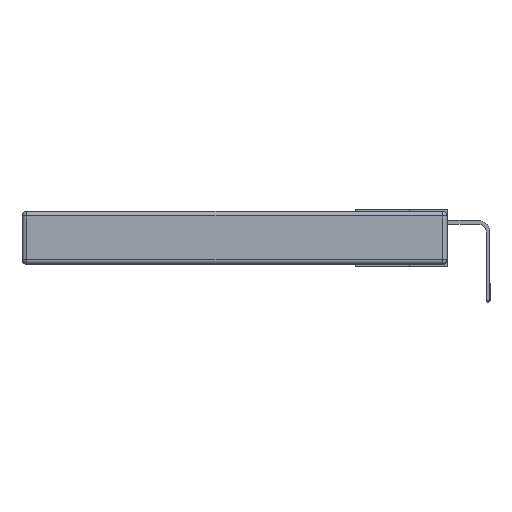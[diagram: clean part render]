
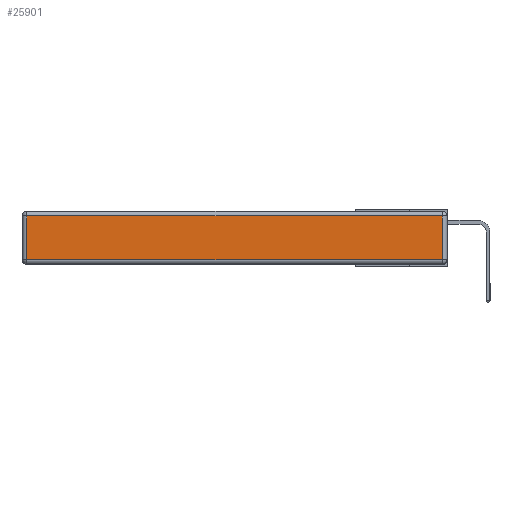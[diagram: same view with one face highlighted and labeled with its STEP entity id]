
A CAD part, left-side view. The second image highlights one B-rep face of the part: STEP entity #25901.
In plain terms, the highlighted planar face has unit normal (-1, 0, 0).
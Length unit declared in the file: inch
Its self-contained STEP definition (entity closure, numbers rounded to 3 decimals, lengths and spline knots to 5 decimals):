
#17 = EDGE_LOOP ( 'NONE', ( #25695, #3863, #17642, #13371 ) ) ;
#898 = VECTOR ( 'NONE', #26544, 39.37008 ) ;
#928 = VECTOR ( 'NONE', #22394, 39.37008 ) ;
#1292 = EDGE_CURVE ( 'NONE', #3934, #8542, #13863, .T. ) ;
#2066 = LINE ( 'NONE', #24042, #22711 ) ;
#2088 = EDGE_CURVE ( 'NONE', #15736, #11245, #26058, .T. ) ;
#3447 = LINE ( 'NONE', #5384, #11836 ) ;
#3863 = ORIENTED_EDGE ( 'NONE', *, *, #22496, .T. ) ;
#3934 = VERTEX_POINT ( 'NONE', #4725 ) ;
#4725 = CARTESIAN_POINT ( 'NONE',  ( 0., 0.03, -0.03 ) ) ;
#5384 = CARTESIAN_POINT ( 'NONE',  ( 0., 2.72, -0.343 ) ) ;
#7131 = FACE_OUTER_BOUND ( 'NONE', #17, .T. ) ;
#7488 = DIRECTION ( 'NONE',  ( -1., 0., 0. ) ) ;
#8542 = VERTEX_POINT ( 'NONE', #16023 ) ;
#9575 = DIRECTION ( 'NONE',  ( 0., 0., 1. ) ) ;
#11245 = VERTEX_POINT ( 'NONE', #12630 ) ;
#11836 = VECTOR ( 'NONE', #21584, 39.37008 ) ;
#12630 = CARTESIAN_POINT ( 'NONE',  ( 0., 0.03, -0.313 ) ) ;
#13371 = ORIENTED_EDGE ( 'NONE', *, *, #21558, .T. ) ;
#13863 = LINE ( 'NONE', #22581, #928 ) ;
#15736 = VERTEX_POINT ( 'NONE', #22889 ) ;
#16023 = CARTESIAN_POINT ( 'NONE',  ( 0., 2.72, -0.03 ) ) ;
#17642 = ORIENTED_EDGE ( 'NONE', *, *, #1292, .T. ) ;
#17893 = PLANE ( 'NONE',  #24985 ) ;
#19752 = CARTESIAN_POINT ( 'NONE',  ( 0., 0., -0.343 ) ) ;
#21558 = EDGE_CURVE ( 'NONE', #8542, #15736, #3447, .T. ) ;
#21584 = DIRECTION ( 'NONE',  ( 0., 0., -1. ) ) ;
#22394 = DIRECTION ( 'NONE',  ( 0., 1., 0. ) ) ;
#22496 = EDGE_CURVE ( 'NONE', #11245, #3934, #2066, .T. ) ;
#22581 = CARTESIAN_POINT ( 'NONE',  ( 0., 2.75, -0.03 ) ) ;
#22711 = VECTOR ( 'NONE', #26011, 39.37008 ) ;
#22889 = CARTESIAN_POINT ( 'NONE',  ( 0., 2.72, -0.313 ) ) ;
#24042 = CARTESIAN_POINT ( 'NONE',  ( 0., 0.03, -0.343 ) ) ;
#24672 = CARTESIAN_POINT ( 'NONE',  ( 0., 0., -0.313 ) ) ;
#24985 = AXIS2_PLACEMENT_3D ( 'NONE', #19752, #7488, #9575 ) ;
#25695 = ORIENTED_EDGE ( 'NONE', *, *, #2088, .T. ) ;
#25901 = ADVANCED_FACE ( 'NONE', ( #7131 ), #17893, .T. ) ;
#26011 = DIRECTION ( 'NONE',  ( 0., 0., 1. ) ) ;
#26058 = LINE ( 'NONE', #24672, #898 ) ;
#26544 = DIRECTION ( 'NONE',  ( 0., -1., 0. ) ) ;
